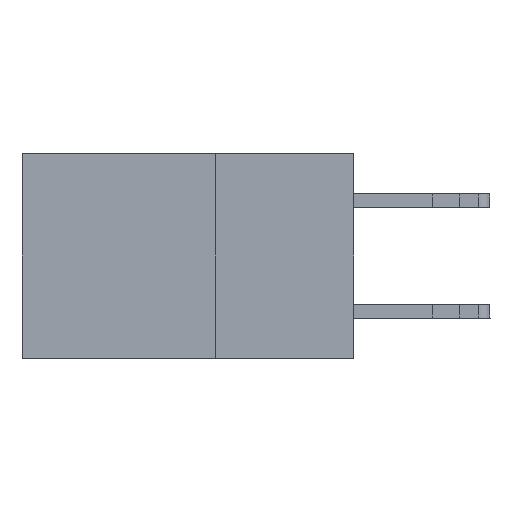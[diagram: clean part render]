
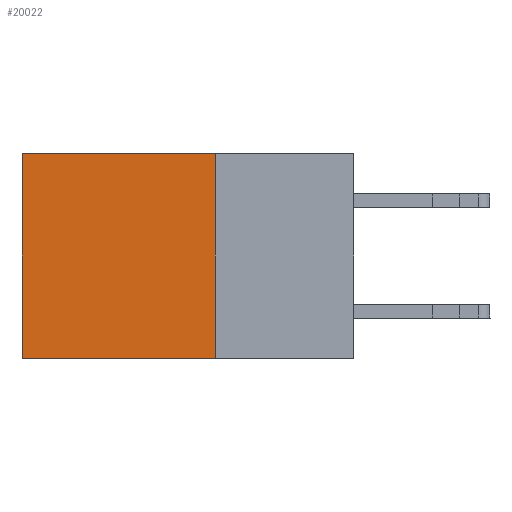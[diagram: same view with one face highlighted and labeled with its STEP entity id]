
A CAD part, left-side view. The second image highlights one B-rep face of the part: STEP entity #20022.
In plain terms, the highlighted planar face has unit normal (-1, 0, 0).
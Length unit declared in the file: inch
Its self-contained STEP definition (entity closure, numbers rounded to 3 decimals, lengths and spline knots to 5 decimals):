
#586 = CARTESIAN_POINT ( 'NONE',  ( 0.2875, 0.25, 0. ) ) ;
#1275 = ORIENTED_EDGE ( 'NONE', *, *, #9160, .T. ) ;
#1382 = LINE ( 'NONE', #20542, #3883 ) ;
#1998 = LINE ( 'NONE', #20157, #20785 ) ;
#2447 = EDGE_LOOP ( 'NONE', ( #1275, #4221, #10893, #9792 ) ) ;
#2925 = VERTEX_POINT ( 'NONE', #8105 ) ;
#3273 = VERTEX_POINT ( 'NONE', #7960 ) ;
#3883 = VECTOR ( 'NONE', #6405, 39.37008 ) ;
#3954 = PLANE ( 'NONE',  #10399 ) ;
#4111 = VERTEX_POINT ( 'NONE', #17878 ) ;
#4221 = ORIENTED_EDGE ( 'NONE', *, *, #17763, .F. ) ;
#5181 = DIRECTION ( 'NONE',  ( 0., 1., 0. ) ) ;
#5382 = VERTEX_POINT ( 'NONE', #8356 ) ;
#5618 = EDGE_CURVE ( 'NONE', #5382, #3273, #1998, .T. ) ;
#5721 = FACE_OUTER_BOUND ( 'NONE', #2447, .T. ) ;
#6405 = DIRECTION ( 'NONE',  ( 0., 0., -1. ) ) ;
#7548 = DIRECTION ( 'NONE',  ( 1., 0., 0. ) ) ;
#7960 = CARTESIAN_POINT ( 'NONE',  ( 0.2875, 0.25, -0.37 ) ) ;
#8076 = DIRECTION ( 'NONE',  ( 0., 0., -1. ) ) ;
#8105 = CARTESIAN_POINT ( 'NONE',  ( 0.2875, 0.6, 0. ) ) ;
#8356 = CARTESIAN_POINT ( 'NONE',  ( 0.2875, 0.25, 0. ) ) ;
#9160 = EDGE_CURVE ( 'NONE', #2925, #4111, #1382, .T. ) ;
#9792 = ORIENTED_EDGE ( 'NONE', *, *, #16317, .T. ) ;
#10399 = AXIS2_PLACEMENT_3D ( 'NONE', #586, #7548, #16893 ) ;
#10893 = ORIENTED_EDGE ( 'NONE', *, *, #5618, .F. ) ;
#12881 = VECTOR ( 'NONE', #21495, 39.37008 ) ;
#13864 = LINE ( 'NONE', #20811, #18018 ) ;
#14544 = CARTESIAN_POINT ( 'NONE',  ( 0.2875, 0.25, 0. ) ) ;
#16317 = EDGE_CURVE ( 'NONE', #5382, #2925, #16376, .T. ) ;
#16376 = LINE ( 'NONE', #14544, #12881 ) ;
#16893 = DIRECTION ( 'NONE',  ( 0., 0., -1. ) ) ;
#17763 = EDGE_CURVE ( 'NONE', #3273, #4111, #13864, .T. ) ;
#17878 = CARTESIAN_POINT ( 'NONE',  ( 0.2875, 0.6, -0.37 ) ) ;
#18018 = VECTOR ( 'NONE', #5181, 39.37008 ) ;
#20022 = ADVANCED_FACE ( 'NONE', ( #5721 ), #3954, .F. ) ;
#20157 = CARTESIAN_POINT ( 'NONE',  ( 0.2875, 0.25, 0. ) ) ;
#20542 = CARTESIAN_POINT ( 'NONE',  ( 0.2875, 0.6, 0. ) ) ;
#20785 = VECTOR ( 'NONE', #8076, 39.37008 ) ;
#20811 = CARTESIAN_POINT ( 'NONE',  ( 0.2875, 0.25, -0.37 ) ) ;
#21495 = DIRECTION ( 'NONE',  ( 0., 1., 0. ) ) ;
